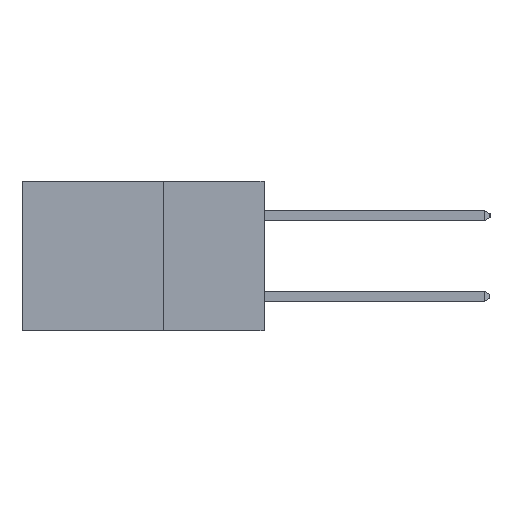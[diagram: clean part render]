
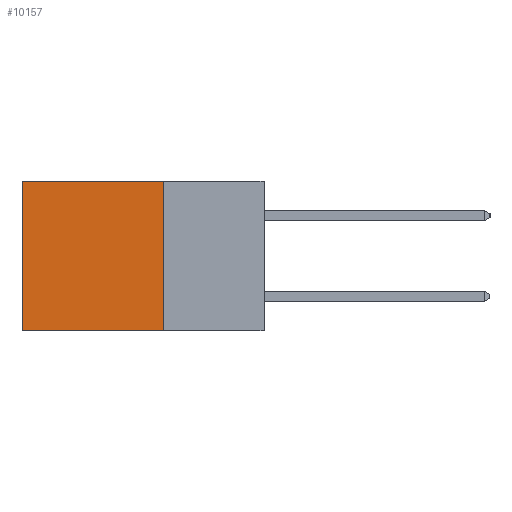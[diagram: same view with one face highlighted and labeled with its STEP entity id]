
A CAD part, left-side view. The second image highlights one B-rep face of the part: STEP entity #10157.
In plain terms, the highlighted planar face has unit normal (-1, 0, 0).
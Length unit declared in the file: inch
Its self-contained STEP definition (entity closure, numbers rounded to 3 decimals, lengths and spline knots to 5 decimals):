
#99 = VECTOR ( 'NONE', #18437, 39.37008 ) ;
#755 = VERTEX_POINT ( 'NONE', #16362 ) ;
#1052 = ORIENTED_EDGE ( 'NONE', *, *, #10101, .F. ) ;
#1511 = DIRECTION ( 'NONE',  ( 0., 1., 0. ) ) ;
#2389 = EDGE_CURVE ( 'NONE', #21045, #755, #19450, .T. ) ;
#2448 = CARTESIAN_POINT ( 'NONE',  ( 0.2615, 0.25, -0.37 ) ) ;
#2496 = EDGE_LOOP ( 'NONE', ( #8119, #12184, #1052, #20810 ) ) ;
#2595 = VERTEX_POINT ( 'NONE', #3152 ) ;
#3152 = CARTESIAN_POINT ( 'NONE',  ( 0.2615, 0.6, 0. ) ) ;
#3779 = EDGE_CURVE ( 'NONE', #2595, #755, #17741, .T. ) ;
#4427 = PLANE ( 'NONE',  #19972 ) ;
#5176 = CARTESIAN_POINT ( 'NONE',  ( 0.2615, 0.25, -0.37 ) ) ;
#6067 = LINE ( 'NONE', #2448, #99 ) ;
#6217 = DIRECTION ( 'NONE',  ( 1., 0., 0. ) ) ;
#6914 = VECTOR ( 'NONE', #1511, 39.37008 ) ;
#8119 = ORIENTED_EDGE ( 'NONE', *, *, #3779, .T. ) ;
#10101 = EDGE_CURVE ( 'NONE', #21589, #21045, #6067, .T. ) ;
#10157 = ADVANCED_FACE ( 'NONE', ( #12727 ), #4427, .F. ) ;
#10394 = CARTESIAN_POINT ( 'NONE',  ( 0.2615, 0.25, 0. ) ) ;
#11892 = DIRECTION ( 'NONE',  ( 0., 1., 0. ) ) ;
#12184 = ORIENTED_EDGE ( 'NONE', *, *, #2389, .F. ) ;
#12727 = FACE_OUTER_BOUND ( 'NONE', #2496, .T. ) ;
#12864 = CARTESIAN_POINT ( 'NONE',  ( 0.2615, 0.25, -0.37 ) ) ;
#13778 = CARTESIAN_POINT ( 'NONE',  ( 0.2615, 0.25, 0. ) ) ;
#16362 = CARTESIAN_POINT ( 'NONE',  ( 0.2615, 0.6, -0.37 ) ) ;
#16832 = CARTESIAN_POINT ( 'NONE',  ( 0.2615, 0.25, -0.37 ) ) ;
#17010 = EDGE_CURVE ( 'NONE', #21589, #2595, #20472, .T. ) ;
#17741 = LINE ( 'NONE', #19241, #20728 ) ;
#18437 = DIRECTION ( 'NONE',  ( 0., 0., -1. ) ) ;
#18510 = DIRECTION ( 'NONE',  ( 0., 0., -1. ) ) ;
#18584 = DIRECTION ( 'NONE',  ( 0., 0., -1. ) ) ;
#19241 = CARTESIAN_POINT ( 'NONE',  ( 0.2615, 0.6, -0.37 ) ) ;
#19450 = LINE ( 'NONE', #12864, #20006 ) ;
#19972 = AXIS2_PLACEMENT_3D ( 'NONE', #16832, #6217, #18584 ) ;
#20006 = VECTOR ( 'NONE', #11892, 39.37008 ) ;
#20472 = LINE ( 'NONE', #10394, #6914 ) ;
#20728 = VECTOR ( 'NONE', #18510, 39.37008 ) ;
#20810 = ORIENTED_EDGE ( 'NONE', *, *, #17010, .T. ) ;
#21045 = VERTEX_POINT ( 'NONE', #5176 ) ;
#21589 = VERTEX_POINT ( 'NONE', #13778 ) ;
